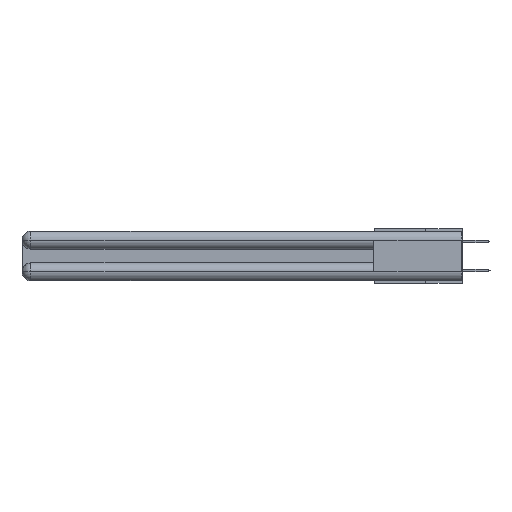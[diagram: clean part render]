
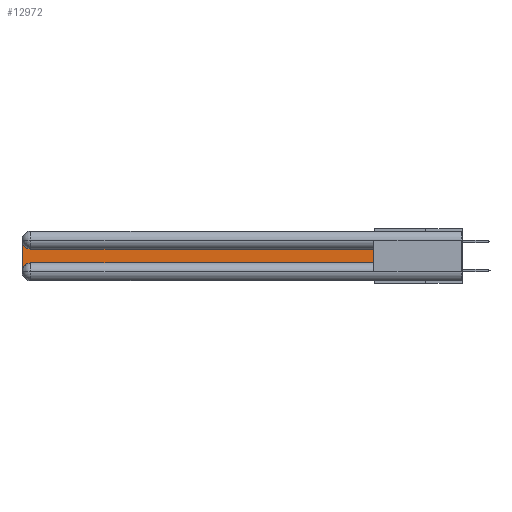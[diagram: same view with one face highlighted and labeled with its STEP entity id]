
A CAD part, left-side view. The second image highlights one B-rep face of the part: STEP entity #12972.
In plain terms, the highlighted planar face has unit normal (-1, 0, 0).
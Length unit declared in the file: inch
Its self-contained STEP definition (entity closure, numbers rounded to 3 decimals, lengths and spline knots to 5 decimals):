
#196 = CARTESIAN_POINT ( 'NONE',  ( 0.075, 0.6, -0.2175 ) ) ;
#363 = CARTESIAN_POINT ( 'NONE',  ( 0.075, 0.6, -0.2175 ) ) ;
#632 = DIRECTION ( 'NONE',  ( 0., 0., -1. ) ) ;
#1414 = EDGE_CURVE ( 'NONE', #13672, #5818, #25955, .T. ) ;
#2274 = EDGE_CURVE ( 'NONE', #22129, #19361, #22714, .T. ) ;
#2524 = EDGE_CURVE ( 'NONE', #19361, #10782, #14196, .T. ) ;
#3109 = CARTESIAN_POINT ( 'NONE',  ( 0.075, 2.94, -0.0625 ) ) ;
#3419 = CIRCLE ( 'NONE', #25898, 0.06 ) ;
#4276 = CARTESIAN_POINT ( 'NONE',  ( 0.075, 2.94, -0.2175 ) ) ;
#4426 = ORIENTED_EDGE ( 'NONE', *, *, #9673, .T. ) ;
#4915 = CARTESIAN_POINT ( 'NONE',  ( 0.075, 3., -0.1225 ) ) ;
#5226 = DIRECTION ( 'NONE',  ( 0., 0., -1. ) ) ;
#5818 = VERTEX_POINT ( 'NONE', #26873 ) ;
#6151 = EDGE_CURVE ( 'NONE', #5818, #22129, #3419, .T. ) ;
#7823 = CARTESIAN_POINT ( 'NONE',  ( 0.075, 3., -0.2175 ) ) ;
#8268 = CARTESIAN_POINT ( 'NONE',  ( 0.075, 0.6, -0.1225 ) ) ;
#8560 = DIRECTION ( 'NONE',  ( 0., 0., -1. ) ) ;
#8748 = AXIS2_PLACEMENT_3D ( 'NONE', #23011, #10535, #8560 ) ;
#8807 = DIRECTION ( 'NONE',  ( 0., -1., 0. ) ) ;
#8897 = PLANE ( 'NONE',  #24945 ) ;
#8987 = DIRECTION ( 'NONE',  ( 1., 0., 0. ) ) ;
#9369 = CARTESIAN_POINT ( 'NONE',  ( 0.075, 0.6, -0.1225 ) ) ;
#9673 = EDGE_CURVE ( 'NONE', #12326, #13672, #11475, .T. ) ;
#10241 = DIRECTION ( 'NONE',  ( 0., 0., 1. ) ) ;
#10396 = DIRECTION ( 'NONE',  ( 0., 1., 0. ) ) ;
#10535 = DIRECTION ( 'NONE',  ( 1., 0., 0. ) ) ;
#10669 = VECTOR ( 'NONE', #10396, 39.37008 ) ;
#10782 = VERTEX_POINT ( 'NONE', #4276 ) ;
#11475 = LINE ( 'NONE', #22704, #12443 ) ;
#12326 = VERTEX_POINT ( 'NONE', #196 ) ;
#12443 = VECTOR ( 'NONE', #10241, 39.37008 ) ;
#12972 = ADVANCED_FACE ( 'NONE', ( #20400 ), #8897, .F. ) ;
#13672 = VERTEX_POINT ( 'NONE', #9369 ) ;
#14196 = CIRCLE ( 'NONE', #8748, 0.06 ) ;
#14248 = VECTOR ( 'NONE', #8807, 39.37008 ) ;
#15234 = CARTESIAN_POINT ( 'NONE',  ( 0.075, 3., -0.2775 ) ) ;
#16115 = DIRECTION ( 'NONE',  ( 0., 0., -1. ) ) ;
#16132 = ORIENTED_EDGE ( 'NONE', *, *, #18579, .T. ) ;
#16785 = ORIENTED_EDGE ( 'NONE', *, *, #2274, .T. ) ;
#17673 = DIRECTION ( 'NONE',  ( 1., 0., 0. ) ) ;
#18579 = EDGE_CURVE ( 'NONE', #10782, #12326, #18895, .T. ) ;
#18895 = LINE ( 'NONE', #363, #14248 ) ;
#19361 = VERTEX_POINT ( 'NONE', #15234 ) ;
#20363 = ORIENTED_EDGE ( 'NONE', *, *, #2524, .T. ) ;
#20400 = FACE_OUTER_BOUND ( 'NONE', #24110, .T. ) ;
#20757 = VECTOR ( 'NONE', #16115, 39.37008 ) ;
#22129 = VERTEX_POINT ( 'NONE', #23534 ) ;
#22704 = CARTESIAN_POINT ( 'NONE',  ( 0.075, 0.6, -0.2175 ) ) ;
#22714 = LINE ( 'NONE', #7823, #20757 ) ;
#23011 = CARTESIAN_POINT ( 'NONE',  ( 0.075, 2.94, -0.2775 ) ) ;
#23534 = CARTESIAN_POINT ( 'NONE',  ( 0.075, 3., -0.0625 ) ) ;
#24110 = EDGE_LOOP ( 'NONE', ( #24922, #26136, #16785, #20363, #16132, #4426 ) ) ;
#24922 = ORIENTED_EDGE ( 'NONE', *, *, #1414, .T. ) ;
#24945 = AXIS2_PLACEMENT_3D ( 'NONE', #4915, #8987, #632 ) ;
#25898 = AXIS2_PLACEMENT_3D ( 'NONE', #3109, #17673, #5226 ) ;
#25955 = LINE ( 'NONE', #8268, #10669 ) ;
#26136 = ORIENTED_EDGE ( 'NONE', *, *, #6151, .T. ) ;
#26873 = CARTESIAN_POINT ( 'NONE',  ( 0.075, 2.94, -0.1225 ) ) ;
